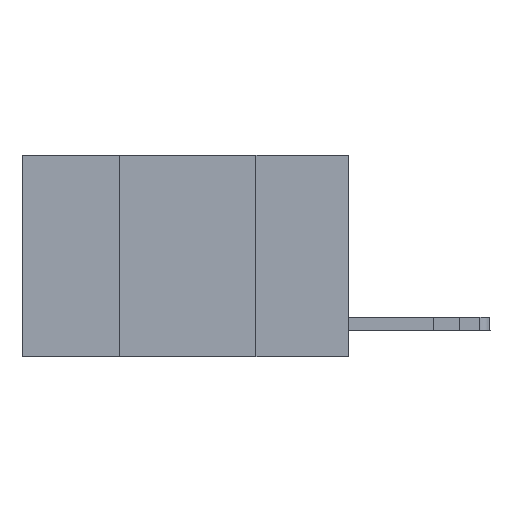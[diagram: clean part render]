
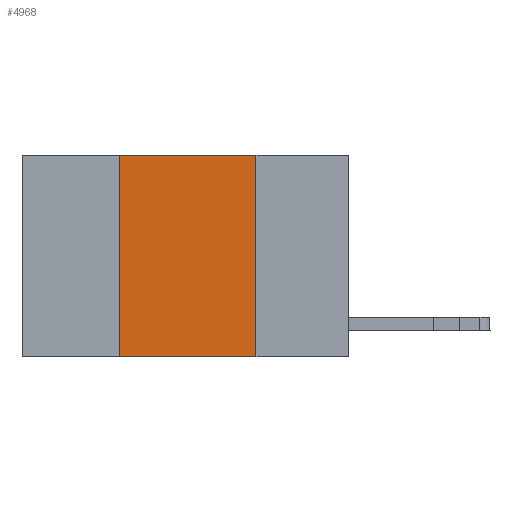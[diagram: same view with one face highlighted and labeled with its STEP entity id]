
A CAD part, left-side view. The second image highlights one B-rep face of the part: STEP entity #4968.
In plain terms, the highlighted planar face has unit normal (-1, 0, 0).
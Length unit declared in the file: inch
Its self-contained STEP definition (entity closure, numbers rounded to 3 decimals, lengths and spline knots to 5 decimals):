
#80 = DIRECTION ( 'NONE',  ( 1., 0., 0. ) ) ;
#334 = DIRECTION ( 'NONE',  ( 0., 0., -1. ) ) ;
#1108 = VERTEX_POINT ( 'NONE', #2575 ) ;
#2328 = ORIENTED_EDGE ( 'NONE', *, *, #11532, .F. ) ;
#2566 = ORIENTED_EDGE ( 'NONE', *, *, #5977, .F. ) ;
#2575 = CARTESIAN_POINT ( 'NONE',  ( 0., 0.42, 0. ) ) ;
#2649 = FACE_OUTER_BOUND ( 'NONE', #11117, .T. ) ;
#2920 = PLANE ( 'NONE',  #16172 ) ;
#3739 = CARTESIAN_POINT ( 'NONE',  ( 0., 0.6, -0.37 ) ) ;
#4036 = DIRECTION ( 'NONE',  ( 0., 0., -1. ) ) ;
#4108 = CARTESIAN_POINT ( 'NONE',  ( 0., 0.6, 0. ) ) ;
#4232 = CARTESIAN_POINT ( 'NONE',  ( 0., 0.42, -0.37 ) ) ;
#4968 = ADVANCED_FACE ( 'NONE', ( #2649 ), #2920, .F. ) ;
#5028 = LINE ( 'NONE', #3739, #10743 ) ;
#5399 = LINE ( 'NONE', #10409, #6877 ) ;
#5704 = VERTEX_POINT ( 'NONE', #14675 ) ;
#5977 = EDGE_CURVE ( 'NONE', #1108, #8110, #6498, .T. ) ;
#6498 = LINE ( 'NONE', #15592, #10858 ) ;
#6877 = VECTOR ( 'NONE', #12034, 39.37008 ) ;
#7874 = LINE ( 'NONE', #13246, #15346 ) ;
#8110 = VERTEX_POINT ( 'NONE', #14908 ) ;
#8249 = ORIENTED_EDGE ( 'NONE', *, *, #9032, .F. ) ;
#8937 = DIRECTION ( 'NONE',  ( 0., -1., 0. ) ) ;
#9032 = EDGE_CURVE ( 'NONE', #12895, #1108, #5399, .T. ) ;
#10409 = CARTESIAN_POINT ( 'NONE',  ( 0., 0.42, 0. ) ) ;
#10743 = VECTOR ( 'NONE', #8937, 39.37008 ) ;
#10858 = VECTOR ( 'NONE', #14140, 39.37008 ) ;
#11117 = EDGE_LOOP ( 'NONE', ( #2328, #2566, #8249, #16474 ) ) ;
#11532 = EDGE_CURVE ( 'NONE', #8110, #5704, #7874, .T. ) ;
#12034 = DIRECTION ( 'NONE',  ( 0., 0., 1. ) ) ;
#12382 = EDGE_CURVE ( 'NONE', #12895, #5704, #5028, .T. ) ;
#12895 = VERTEX_POINT ( 'NONE', #4232 ) ;
#13246 = CARTESIAN_POINT ( 'NONE',  ( 0., 0.17, 0. ) ) ;
#14140 = DIRECTION ( 'NONE',  ( 0., -1., 0. ) ) ;
#14675 = CARTESIAN_POINT ( 'NONE',  ( 0., 0.17, -0.37 ) ) ;
#14908 = CARTESIAN_POINT ( 'NONE',  ( 0., 0.17, 0. ) ) ;
#15346 = VECTOR ( 'NONE', #4036, 39.37008 ) ;
#15592 = CARTESIAN_POINT ( 'NONE',  ( 0., 0.6, 0. ) ) ;
#16172 = AXIS2_PLACEMENT_3D ( 'NONE', #4108, #80, #334 ) ;
#16474 = ORIENTED_EDGE ( 'NONE', *, *, #12382, .T. ) ;
